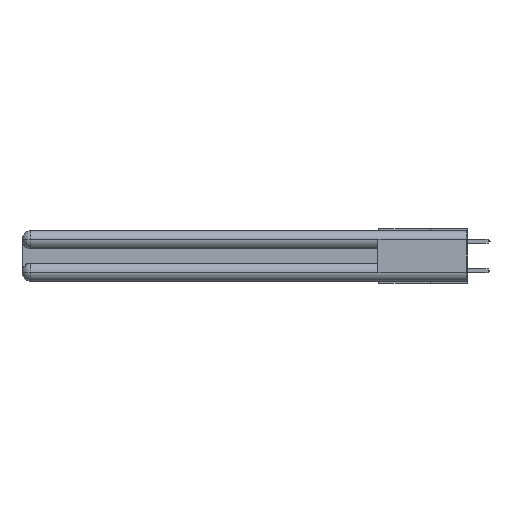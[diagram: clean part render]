
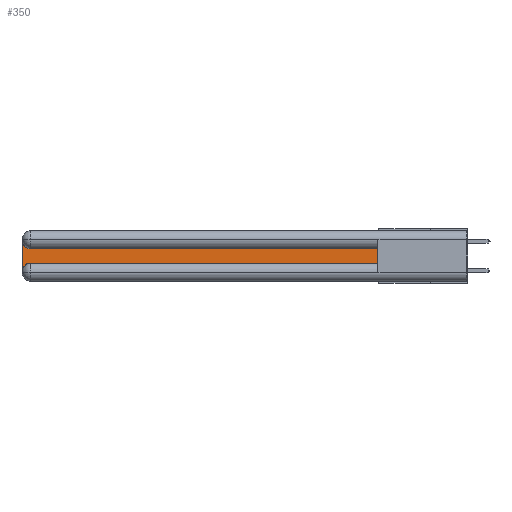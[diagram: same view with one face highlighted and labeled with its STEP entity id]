
A CAD part, left-side view. The second image highlights one B-rep face of the part: STEP entity #350.
In plain terms, the highlighted planar face has unit normal (-1, 0, 0).
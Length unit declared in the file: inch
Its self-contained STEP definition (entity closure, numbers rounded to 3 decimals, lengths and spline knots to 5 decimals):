
#128 = VERTEX_POINT ( 'NONE', #12859 ) ;
#350 = ADVANCED_FACE ( 'NONE', ( #11592 ), #25649, .F. ) ;
#884 = ORIENTED_EDGE ( 'NONE', *, *, #9500, .T. ) ;
#1203 = DIRECTION ( 'NONE',  ( 0., 0., -1. ) ) ;
#1981 = CARTESIAN_POINT ( 'NONE',  ( 0.075, 2.94, -0.1225 ) ) ;
#3209 = CARTESIAN_POINT ( 'NONE',  ( 0.075, 0.6, -0.2175 ) ) ;
#3681 = DIRECTION ( 'NONE',  ( 0., 0., -1. ) ) ;
#4235 = EDGE_CURVE ( 'NONE', #6151, #13328, #23833, .T. ) ;
#4545 = CARTESIAN_POINT ( 'NONE',  ( 0.075, 2.94, -0.2175 ) ) ;
#5304 = LINE ( 'NONE', #21202, #7573 ) ;
#5320 = EDGE_CURVE ( 'NONE', #13328, #13023, #12357, .T. ) ;
#5673 = EDGE_CURVE ( 'NONE', #13023, #128, #11929, .T. ) ;
#5693 = DIRECTION ( 'NONE',  ( 0., -1., 0. ) ) ;
#6151 = VERTEX_POINT ( 'NONE', #13318 ) ;
#6256 = VECTOR ( 'NONE', #5693, 39.37008 ) ;
#7573 = VECTOR ( 'NONE', #31322, 39.37008 ) ;
#8680 = CARTESIAN_POINT ( 'NONE',  ( 0.075, 2.94, -0.0625 ) ) ;
#8850 = DIRECTION ( 'NONE',  ( 0., 0., -1. ) ) ;
#9500 = EDGE_CURVE ( 'NONE', #16570, #21764, #16480, .T. ) ;
#10629 = CARTESIAN_POINT ( 'NONE',  ( 0.075, 0.6, -0.2175 ) ) ;
#10737 = DIRECTION ( 'NONE',  ( 0., 0., 1. ) ) ;
#11592 = FACE_OUTER_BOUND ( 'NONE', #17317, .T. ) ;
#11929 = LINE ( 'NONE', #10629, #17201 ) ;
#12357 = LINE ( 'NONE', #28808, #6256 ) ;
#12859 = CARTESIAN_POINT ( 'NONE',  ( 0.075, 0.6, -0.1225 ) ) ;
#13023 = VERTEX_POINT ( 'NONE', #3209 ) ;
#13318 = CARTESIAN_POINT ( 'NONE',  ( 0.075, 3., -0.2775 ) ) ;
#13328 = VERTEX_POINT ( 'NONE', #4545 ) ;
#16480 = CIRCLE ( 'NONE', #30531, 0.06 ) ;
#16570 = VERTEX_POINT ( 'NONE', #1981 ) ;
#16635 = CARTESIAN_POINT ( 'NONE',  ( 0.075, 0.6, -0.1225 ) ) ;
#17049 = LINE ( 'NONE', #16635, #18250 ) ;
#17201 = VECTOR ( 'NONE', #10737, 39.37008 ) ;
#17317 = EDGE_LOOP ( 'NONE', ( #24132, #884, #25549, #27774, #20479, #20540 ) ) ;
#18250 = VECTOR ( 'NONE', #28647, 39.37008 ) ;
#20186 = CARTESIAN_POINT ( 'NONE',  ( 0.075, 3., -0.0625 ) ) ;
#20479 = ORIENTED_EDGE ( 'NONE', *, *, #5320, .T. ) ;
#20540 = ORIENTED_EDGE ( 'NONE', *, *, #5673, .T. ) ;
#20721 = EDGE_CURVE ( 'NONE', #21764, #6151, #5304, .T. ) ;
#21095 = CARTESIAN_POINT ( 'NONE',  ( 0.075, 3., -0.1225 ) ) ;
#21202 = CARTESIAN_POINT ( 'NONE',  ( 0.075, 3., -0.2175 ) ) ;
#21764 = VERTEX_POINT ( 'NONE', #20186 ) ;
#23555 = CARTESIAN_POINT ( 'NONE',  ( 0.075, 2.94, -0.2775 ) ) ;
#23833 = CIRCLE ( 'NONE', #24731, 0.06 ) ;
#24132 = ORIENTED_EDGE ( 'NONE', *, *, #26803, .T. ) ;
#24731 = AXIS2_PLACEMENT_3D ( 'NONE', #23555, #25965, #3681 ) ;
#25549 = ORIENTED_EDGE ( 'NONE', *, *, #20721, .T. ) ;
#25649 = PLANE ( 'NONE',  #30570 ) ;
#25965 = DIRECTION ( 'NONE',  ( 1., 0., 0. ) ) ;
#26803 = EDGE_CURVE ( 'NONE', #128, #16570, #17049, .T. ) ;
#27774 = ORIENTED_EDGE ( 'NONE', *, *, #4235, .T. ) ;
#28184 = DIRECTION ( 'NONE',  ( 1., 0., 0. ) ) ;
#28647 = DIRECTION ( 'NONE',  ( 0., 1., 0. ) ) ;
#28808 = CARTESIAN_POINT ( 'NONE',  ( 0.075, 0.6, -0.2175 ) ) ;
#30340 = DIRECTION ( 'NONE',  ( 1., 0., 0. ) ) ;
#30531 = AXIS2_PLACEMENT_3D ( 'NONE', #8680, #30340, #1203 ) ;
#30570 = AXIS2_PLACEMENT_3D ( 'NONE', #21095, #28184, #8850 ) ;
#31322 = DIRECTION ( 'NONE',  ( 0., 0., -1. ) ) ;
